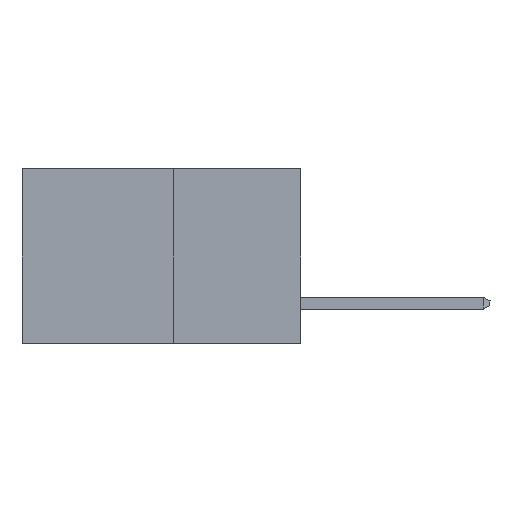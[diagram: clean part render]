
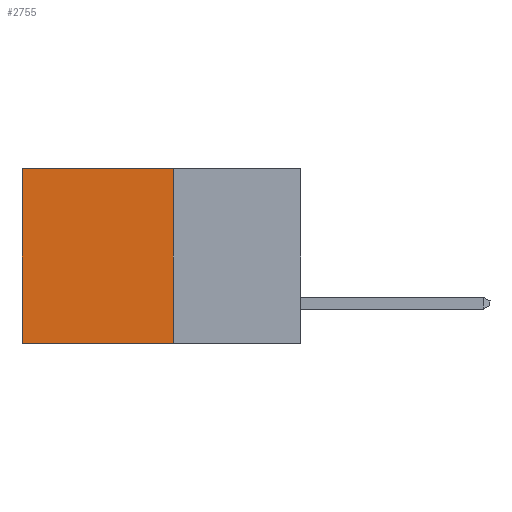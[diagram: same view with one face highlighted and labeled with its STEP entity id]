
A CAD part, left-side view. The second image highlights one B-rep face of the part: STEP entity #2755.
In plain terms, the highlighted planar face has unit normal (-1, 0, 0).
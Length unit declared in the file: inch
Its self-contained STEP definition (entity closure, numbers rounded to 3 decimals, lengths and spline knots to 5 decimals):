
#319 = DIRECTION ( 'NONE',  ( 0., 0., -1. ) ) ;
#523 = VECTOR ( 'NONE', #8005, 39.37008 ) ;
#929 = EDGE_CURVE ( 'NONE', #14625, #24232, #21134, .T. ) ;
#1152 = VECTOR ( 'NONE', #31582, 39.37008 ) ;
#2351 = DIRECTION ( 'NONE',  ( 0., 1., 0. ) ) ;
#2755 = ADVANCED_FACE ( 'NONE', ( #10170 ), #3497, .F. ) ;
#3456 = DIRECTION ( 'NONE',  ( 1., 0., 0. ) ) ;
#3497 = PLANE ( 'NONE',  #8280 ) ;
#3530 = DIRECTION ( 'NONE',  ( 0., 0., -1. ) ) ;
#5953 = CARTESIAN_POINT ( 'NONE',  ( 0.277, 0.27, -0.37 ) ) ;
#6841 = VECTOR ( 'NONE', #2351, 39.37008 ) ;
#8005 = DIRECTION ( 'NONE',  ( 0., 1., 0. ) ) ;
#8280 = AXIS2_PLACEMENT_3D ( 'NONE', #20144, #3456, #3530 ) ;
#8372 = ORIENTED_EDGE ( 'NONE', *, *, #29630, .F. ) ;
#9103 = VERTEX_POINT ( 'NONE', #5953 ) ;
#10170 = FACE_OUTER_BOUND ( 'NONE', #29994, .T. ) ;
#10720 = CARTESIAN_POINT ( 'NONE',  ( 0.277, 0.59, -0.37 ) ) ;
#10744 = VECTOR ( 'NONE', #319, 39.37008 ) ;
#13786 = LINE ( 'NONE', #30550, #6841 ) ;
#14625 = VERTEX_POINT ( 'NONE', #20329 ) ;
#15716 = ORIENTED_EDGE ( 'NONE', *, *, #929, .T. ) ;
#16296 = ORIENTED_EDGE ( 'NONE', *, *, #27076, .T. ) ;
#16361 = CARTESIAN_POINT ( 'NONE',  ( 0.277, 0.27, -0.37 ) ) ;
#17613 = VERTEX_POINT ( 'NONE', #27727 ) ;
#19512 = CARTESIAN_POINT ( 'NONE',  ( 0.277, 0.27, 0. ) ) ;
#20144 = CARTESIAN_POINT ( 'NONE',  ( 0.277, 0.27, -0.37 ) ) ;
#20329 = CARTESIAN_POINT ( 'NONE',  ( 0.277, 0.27, 0. ) ) ;
#20976 = LINE ( 'NONE', #16361, #1152 ) ;
#21134 = LINE ( 'NONE', #19512, #523 ) ;
#24232 = VERTEX_POINT ( 'NONE', #25251 ) ;
#24314 = EDGE_CURVE ( 'NONE', #9103, #17613, #13786, .T. ) ;
#25004 = ORIENTED_EDGE ( 'NONE', *, *, #24314, .F. ) ;
#25251 = CARTESIAN_POINT ( 'NONE',  ( 0.277, 0.59, 0. ) ) ;
#27076 = EDGE_CURVE ( 'NONE', #24232, #17613, #32669, .T. ) ;
#27727 = CARTESIAN_POINT ( 'NONE',  ( 0.277, 0.59, -0.37 ) ) ;
#29630 = EDGE_CURVE ( 'NONE', #14625, #9103, #20976, .T. ) ;
#29994 = EDGE_LOOP ( 'NONE', ( #16296, #25004, #8372, #15716 ) ) ;
#30550 = CARTESIAN_POINT ( 'NONE',  ( 0.277, 0.27, -0.37 ) ) ;
#31582 = DIRECTION ( 'NONE',  ( 0., 0., -1. ) ) ;
#32669 = LINE ( 'NONE', #10720, #10744 ) ;
